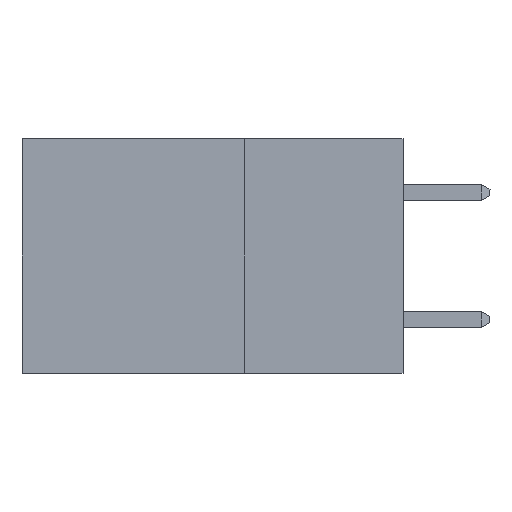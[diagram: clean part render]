
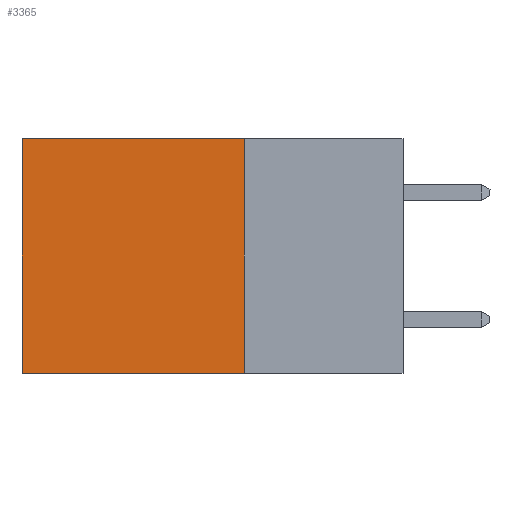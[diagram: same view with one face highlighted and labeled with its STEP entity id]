
A CAD part, left-side view. The second image highlights one B-rep face of the part: STEP entity #3365.
In plain terms, the highlighted planar face has unit normal (-1, 0, 0).
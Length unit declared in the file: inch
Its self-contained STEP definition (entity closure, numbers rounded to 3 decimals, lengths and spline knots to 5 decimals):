
#347 = VERTEX_POINT ( 'NONE', #2050 ) ;
#891 = CARTESIAN_POINT ( 'NONE',  ( 0.2875, 0.25, 0. ) ) ;
#1212 = LINE ( 'NONE', #891, #8531 ) ;
#1326 = CARTESIAN_POINT ( 'NONE',  ( 0.2875, 0.25, 0. ) ) ;
#1640 = CARTESIAN_POINT ( 'NONE',  ( 0.2875, 0.6, -0.37 ) ) ;
#1819 = LINE ( 'NONE', #4154, #4132 ) ;
#2050 = CARTESIAN_POINT ( 'NONE',  ( 0.2875, 0.25, -0.37 ) ) ;
#2222 = EDGE_CURVE ( 'NONE', #5255, #3487, #8478, .T. ) ;
#2831 = PLANE ( 'NONE',  #6940 ) ;
#2922 = ORIENTED_EDGE ( 'NONE', *, *, #5952, .T. ) ;
#3365 = ADVANCED_FACE ( 'NONE', ( #6110 ), #2831, .F. ) ;
#3383 = VECTOR ( 'NONE', #4257, 39.37008 ) ;
#3487 = VERTEX_POINT ( 'NONE', #9563 ) ;
#3633 = LINE ( 'NONE', #7261, #3383 ) ;
#3886 = DIRECTION ( 'NONE',  ( 0., 0., -1. ) ) ;
#4132 = VECTOR ( 'NONE', #4186, 39.37008 ) ;
#4135 = CARTESIAN_POINT ( 'NONE',  ( 0.2875, 0.25, 0. ) ) ;
#4154 = CARTESIAN_POINT ( 'NONE',  ( 0.2875, 0.6, 0. ) ) ;
#4186 = DIRECTION ( 'NONE',  ( 0., 0., -1. ) ) ;
#4257 = DIRECTION ( 'NONE',  ( 0., 1., 0. ) ) ;
#4329 = VECTOR ( 'NONE', #9607, 39.37008 ) ;
#4462 = DIRECTION ( 'NONE',  ( 1., 0., 0. ) ) ;
#5255 = VERTEX_POINT ( 'NONE', #5812 ) ;
#5375 = EDGE_LOOP ( 'NONE', ( #2922, #7632, #6139, #9250 ) ) ;
#5429 = EDGE_CURVE ( 'NONE', #5255, #347, #1212, .T. ) ;
#5812 = CARTESIAN_POINT ( 'NONE',  ( 0.2875, 0.25, 0. ) ) ;
#5952 = EDGE_CURVE ( 'NONE', #3487, #8533, #1819, .T. ) ;
#6110 = FACE_OUTER_BOUND ( 'NONE', #5375, .T. ) ;
#6139 = ORIENTED_EDGE ( 'NONE', *, *, #5429, .F. ) ;
#6940 = AXIS2_PLACEMENT_3D ( 'NONE', #1326, #4462, #7446 ) ;
#7261 = CARTESIAN_POINT ( 'NONE',  ( 0.2875, 0.25, -0.37 ) ) ;
#7446 = DIRECTION ( 'NONE',  ( 0., 0., -1. ) ) ;
#7632 = ORIENTED_EDGE ( 'NONE', *, *, #8643, .F. ) ;
#8478 = LINE ( 'NONE', #4135, #4329 ) ;
#8531 = VECTOR ( 'NONE', #3886, 39.37008 ) ;
#8533 = VERTEX_POINT ( 'NONE', #1640 ) ;
#8643 = EDGE_CURVE ( 'NONE', #347, #8533, #3633, .T. ) ;
#9250 = ORIENTED_EDGE ( 'NONE', *, *, #2222, .T. ) ;
#9563 = CARTESIAN_POINT ( 'NONE',  ( 0.2875, 0.6, 0. ) ) ;
#9607 = DIRECTION ( 'NONE',  ( 0., 1., 0. ) ) ;
